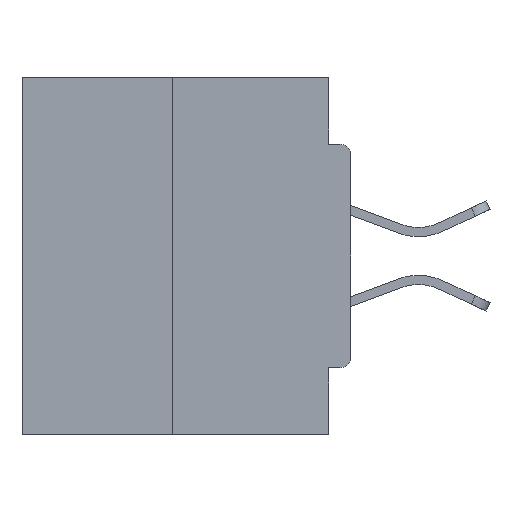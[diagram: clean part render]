
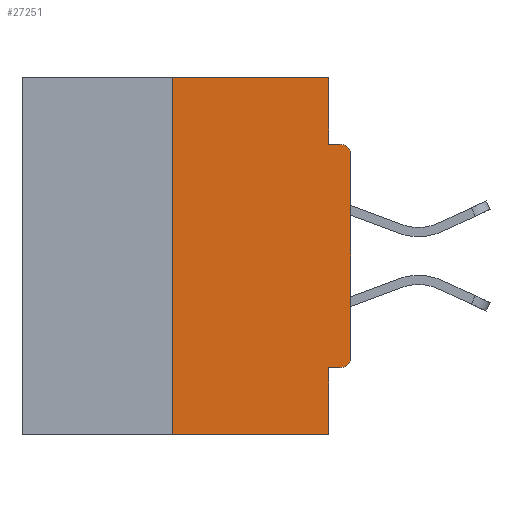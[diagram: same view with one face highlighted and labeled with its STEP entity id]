
A CAD part, left-side view. The second image highlights one B-rep face of the part: STEP entity #27251.
In plain terms, the highlighted planar face has unit normal (-1, 0, 0).
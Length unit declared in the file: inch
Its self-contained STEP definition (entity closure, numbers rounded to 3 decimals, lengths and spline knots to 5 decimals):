
#32 = CARTESIAN_POINT ( 'NONE',  ( 0., 0.031, -0.5 ) ) ;
#152 = VECTOR ( 'NONE', #27390, 39.37008 ) ;
#1407 = VERTEX_POINT ( 'NONE', #32 ) ;
#1668 = CARTESIAN_POINT ( 'NONE',  ( 0., 0.46, 0. ) ) ;
#1794 = LINE ( 'NONE', #5578, #15736 ) ;
#2023 = LINE ( 'NONE', #27876, #6678 ) ;
#2420 = DIRECTION ( 'NONE',  ( -1., 0., 0. ) ) ;
#3114 = VECTOR ( 'NONE', #35507, 39.37008 ) ;
#3598 = LINE ( 'NONE', #27604, #17560 ) ;
#3859 = AXIS2_PLACEMENT_3D ( 'NONE', #42011, #2420, #38839 ) ;
#5047 = EDGE_LOOP ( 'NONE', ( #5847, #29527, #18451, #22559, #19184, #38976, #38064, #42088, #39582, #18760 ) ) ;
#5155 = EDGE_CURVE ( 'NONE', #42809, #6241, #8327, .T. ) ;
#5578 = CARTESIAN_POINT ( 'NONE',  ( 0., 0.25, 0. ) ) ;
#5828 = CARTESIAN_POINT ( 'NONE',  ( 0., 0.031, -0.0935 ) ) ;
#5847 = ORIENTED_EDGE ( 'NONE', *, *, #19112, .F. ) ;
#6241 = VERTEX_POINT ( 'NONE', #40973 ) ;
#6618 = VERTEX_POINT ( 'NONE', #5828 ) ;
#6678 = VECTOR ( 'NONE', #15483, 39.37008 ) ;
#7016 = LINE ( 'NONE', #38159, #11668 ) ;
#7751 = CARTESIAN_POINT ( 'NONE',  ( 0., 0., 0. ) ) ;
#8327 = CIRCLE ( 'NONE', #3859, 0.015 ) ;
#8575 = CARTESIAN_POINT ( 'NONE',  ( 0., 0.031, -0.4065 ) ) ;
#11668 = VECTOR ( 'NONE', #18368, 39.37008 ) ;
#11786 = DIRECTION ( 'NONE',  ( 0., -1., 0. ) ) ;
#12869 = VECTOR ( 'NONE', #25771, 39.37008 ) ;
#13562 = CARTESIAN_POINT ( 'NONE',  ( 0., 0.031, 0. ) ) ;
#14272 = VERTEX_POINT ( 'NONE', #35427 ) ;
#14613 = AXIS2_PLACEMENT_3D ( 'NONE', #36151, #30076, #33126 ) ;
#15302 = CARTESIAN_POINT ( 'NONE',  ( 0., 0.031, 0. ) ) ;
#15483 = DIRECTION ( 'NONE',  ( 0., -1., 0. ) ) ;
#15736 = VECTOR ( 'NONE', #32028, 39.37008 ) ;
#16480 = CARTESIAN_POINT ( 'NONE',  ( 0., 0.015, -0.0935 ) ) ;
#16694 = LINE ( 'NONE', #1668, #17208 ) ;
#17208 = VECTOR ( 'NONE', #11786, 39.37008 ) ;
#17560 = VECTOR ( 'NONE', #24135, 39.37008 ) ;
#18368 = DIRECTION ( 'NONE',  ( 0., 1., 0. ) ) ;
#18451 = ORIENTED_EDGE ( 'NONE', *, *, #38712, .T. ) ;
#18760 = ORIENTED_EDGE ( 'NONE', *, *, #25370, .F. ) ;
#18937 = PLANE ( 'NONE',  #19742 ) ;
#19084 = DIRECTION ( 'NONE',  ( 1., 0., 0. ) ) ;
#19112 = EDGE_CURVE ( 'NONE', #24458, #40197, #16694, .T. ) ;
#19184 = ORIENTED_EDGE ( 'NONE', *, *, #30947, .F. ) ;
#19344 = EDGE_CURVE ( 'NONE', #6241, #14272, #39469, .T. ) ;
#19742 = AXIS2_PLACEMENT_3D ( 'NONE', #29494, #19084, #32398 ) ;
#20121 = LINE ( 'NONE', #32705, #12869 ) ;
#22476 = EDGE_CURVE ( 'NONE', #14272, #38975, #28325, .T. ) ;
#22559 = ORIENTED_EDGE ( 'NONE', *, *, #33889, .F. ) ;
#22790 = LINE ( 'NONE', #15302, #3114 ) ;
#24135 = DIRECTION ( 'NONE',  ( 0., -1., 0. ) ) ;
#24458 = VERTEX_POINT ( 'NONE', #28975 ) ;
#25370 = EDGE_CURVE ( 'NONE', #40197, #6618, #22790, .T. ) ;
#25771 = DIRECTION ( 'NONE',  ( 0., 0., -1. ) ) ;
#27251 = ADVANCED_FACE ( 'NONE', ( #30437 ), #18937, .F. ) ;
#27263 = CARTESIAN_POINT ( 'NONE',  ( 0., 0.015, -0.4065 ) ) ;
#27390 = DIRECTION ( 'NONE',  ( 0., 0., 1. ) ) ;
#27604 = CARTESIAN_POINT ( 'NONE',  ( 0., 0.46, -0.5 ) ) ;
#27876 = CARTESIAN_POINT ( 'NONE',  ( 0., 0., -0.0935 ) ) ;
#28325 = CIRCLE ( 'NONE', #14613, 0.015 ) ;
#28975 = CARTESIAN_POINT ( 'NONE',  ( 0., 0.25, 0. ) ) ;
#29494 = CARTESIAN_POINT ( 'NONE',  ( 0., 0.46, 0. ) ) ;
#29527 = ORIENTED_EDGE ( 'NONE', *, *, #31706, .F. ) ;
#30076 = DIRECTION ( 'NONE',  ( -1., 0., 0. ) ) ;
#30437 = FACE_OUTER_BOUND ( 'NONE', #5047, .T. ) ;
#30947 = EDGE_CURVE ( 'NONE', #42809, #40803, #7016, .T. ) ;
#31706 = EDGE_CURVE ( 'NONE', #34812, #24458, #1794, .T. ) ;
#32028 = DIRECTION ( 'NONE',  ( 0., 0., 1. ) ) ;
#32398 = DIRECTION ( 'NONE',  ( 0., 0., -1. ) ) ;
#32705 = CARTESIAN_POINT ( 'NONE',  ( 0., 0.031, -0.5 ) ) ;
#33126 = DIRECTION ( 'NONE',  ( 0., 0., -1. ) ) ;
#33889 = EDGE_CURVE ( 'NONE', #40803, #1407, #20121, .T. ) ;
#34387 = CARTESIAN_POINT ( 'NONE',  ( 0., 0.25, -0.5 ) ) ;
#34812 = VERTEX_POINT ( 'NONE', #34387 ) ;
#35427 = CARTESIAN_POINT ( 'NONE',  ( 0., 0., -0.1085 ) ) ;
#35507 = DIRECTION ( 'NONE',  ( 0., 0., -1. ) ) ;
#36151 = CARTESIAN_POINT ( 'NONE',  ( 0., 0.015, -0.1085 ) ) ;
#38064 = ORIENTED_EDGE ( 'NONE', *, *, #19344, .T. ) ;
#38159 = CARTESIAN_POINT ( 'NONE',  ( 0., 0., -0.4065 ) ) ;
#38712 = EDGE_CURVE ( 'NONE', #34812, #1407, #3598, .T. ) ;
#38839 = DIRECTION ( 'NONE',  ( 0., 0., -1. ) ) ;
#38901 = EDGE_CURVE ( 'NONE', #6618, #38975, #2023, .T. ) ;
#38975 = VERTEX_POINT ( 'NONE', #16480 ) ;
#38976 = ORIENTED_EDGE ( 'NONE', *, *, #5155, .T. ) ;
#39469 = LINE ( 'NONE', #7751, #152 ) ;
#39582 = ORIENTED_EDGE ( 'NONE', *, *, #38901, .F. ) ;
#40197 = VERTEX_POINT ( 'NONE', #13562 ) ;
#40803 = VERTEX_POINT ( 'NONE', #8575 ) ;
#40973 = CARTESIAN_POINT ( 'NONE',  ( 0., 0., -0.3915 ) ) ;
#42011 = CARTESIAN_POINT ( 'NONE',  ( 0., 0.015, -0.3915 ) ) ;
#42088 = ORIENTED_EDGE ( 'NONE', *, *, #22476, .T. ) ;
#42809 = VERTEX_POINT ( 'NONE', #27263 ) ;
